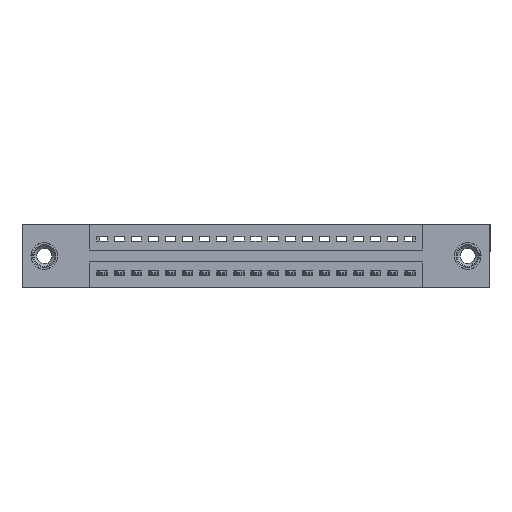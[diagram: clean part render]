
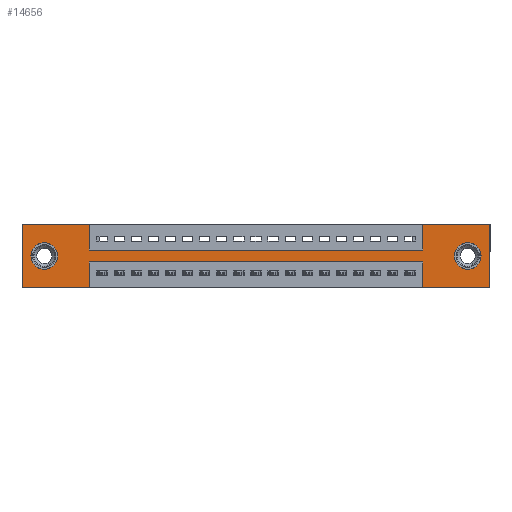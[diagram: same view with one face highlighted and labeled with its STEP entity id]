
A CAD part, front view. The second image highlights one B-rep face of the part: STEP entity #14656.
In plain terms, the highlighted planar face has unit normal (0, -1, 0).
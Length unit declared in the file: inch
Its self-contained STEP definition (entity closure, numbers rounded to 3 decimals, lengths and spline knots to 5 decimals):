
#80 = CARTESIAN_POINT ( 'NONE',  ( 0., 0., 0. ) ) ;
#273 = EDGE_CURVE ( 'NONE', #2156, #12889, #7085, .T. ) ;
#484 = ORIENTED_EDGE ( 'NONE', *, *, #7590, .F. ) ;
#587 = VECTOR ( 'NONE', #12232, 39.37008 ) ;
#705 = AXIS2_PLACEMENT_3D ( 'NONE', #14344, #5183, #9753 ) ;
#764 = CARTESIAN_POINT ( 'NONE',  ( 0.13, 0., -0.107 ) ) ;
#942 = VECTOR ( 'NONE', #14525, 39.37008 ) ;
#1250 = VECTOR ( 'NONE', #10655, 39.37008 ) ;
#1384 = CARTESIAN_POINT ( 'NONE',  ( 0.13, 0., -0.185 ) ) ;
#1507 = DIRECTION ( 'NONE',  ( 0., 1., 0. ) ) ;
#1546 = CARTESIAN_POINT ( 'NONE',  ( 0., 0., 0. ) ) ;
#1568 = ORIENTED_EDGE ( 'NONE', *, *, #5606, .F. ) ;
#1575 = ORIENTED_EDGE ( 'NONE', *, *, #3872, .F. ) ;
#1756 = ORIENTED_EDGE ( 'NONE', *, *, #2235, .T. ) ;
#1924 = CARTESIAN_POINT ( 'NONE',  ( 0.3925, 0., 0. ) ) ;
#1944 = VERTEX_POINT ( 'NONE', #3191 ) ;
#1962 = ORIENTED_EDGE ( 'NONE', *, *, #273, .F. ) ;
#2027 = LINE ( 'NONE', #11037, #2690 ) ;
#2156 = VERTEX_POINT ( 'NONE', #8819 ) ;
#2235 = EDGE_CURVE ( 'NONE', #10011, #6532, #18447, .T. ) ;
#2266 = FACE_BOUND ( 'NONE', #15954, .T. ) ;
#2497 = EDGE_LOOP ( 'NONE', ( #3591, #1756 ) ) ;
#2690 = VECTOR ( 'NONE', #15752, 39.37008 ) ;
#2843 = CARTESIAN_POINT ( 'NONE',  ( 0.13, 0., -0.263 ) ) ;
#3062 = DIRECTION ( 'NONE',  ( 0., 0., -1. ) ) ;
#3191 = CARTESIAN_POINT ( 'NONE',  ( 2.3425, 0., -0.37 ) ) ;
#3228 = LINE ( 'NONE', #9522, #13664 ) ;
#3409 = CARTESIAN_POINT ( 'NONE',  ( 0., 0., 0. ) ) ;
#3501 = CARTESIAN_POINT ( 'NONE',  ( 0.3925, 0., -0.22 ) ) ;
#3530 = DIRECTION ( 'NONE',  ( 0., 0., -1. ) ) ;
#3554 = CARTESIAN_POINT ( 'NONE',  ( 2.3425, 0., -0.22 ) ) ;
#3591 = ORIENTED_EDGE ( 'NONE', *, *, #18107, .T. ) ;
#3616 = ORIENTED_EDGE ( 'NONE', *, *, #11056, .F. ) ;
#3793 = AXIS2_PLACEMENT_3D ( 'NONE', #13927, #7788, #18443 ) ;
#3868 = LINE ( 'NONE', #17785, #5732 ) ;
#3872 = EDGE_CURVE ( 'NONE', #16847, #8612, #2027, .T. ) ;
#4174 = EDGE_CURVE ( 'NONE', #12920, #9953, #19240, .T. ) ;
#4819 = DIRECTION ( 'NONE',  ( -1., 0., 0. ) ) ;
#5183 = DIRECTION ( 'NONE',  ( 0., 1., 0. ) ) ;
#5366 = CARTESIAN_POINT ( 'NONE',  ( 2.735, 0., 0. ) ) ;
#5381 = VERTEX_POINT ( 'NONE', #764 ) ;
#5606 = EDGE_CURVE ( 'NONE', #9953, #2156, #18766, .T. ) ;
#5732 = VECTOR ( 'NONE', #19276, 39.37008 ) ;
#5865 = VECTOR ( 'NONE', #8054, 39.37008 ) ;
#5976 = CIRCLE ( 'NONE', #3793, 0.078 ) ;
#5977 = VECTOR ( 'NONE', #3062, 39.37008 ) ;
#5986 = VERTEX_POINT ( 'NONE', #2843 ) ;
#6260 = VECTOR ( 'NONE', #3530, 39.37008 ) ;
#6328 = EDGE_CURVE ( 'NONE', #5986, #5381, #8030, .T. ) ;
#6339 = LINE ( 'NONE', #18823, #10898 ) ;
#6477 = VERTEX_POINT ( 'NONE', #8709 ) ;
#6479 = ORIENTED_EDGE ( 'NONE', *, *, #13541, .F. ) ;
#6532 = VERTEX_POINT ( 'NONE', #10853 ) ;
#6617 = AXIS2_PLACEMENT_3D ( 'NONE', #16833, #10727, #10925 ) ;
#6768 = CIRCLE ( 'NONE', #705, 0.078 ) ;
#6853 = CARTESIAN_POINT ( 'NONE',  ( 2.735, 0., -0.37 ) ) ;
#7085 = LINE ( 'NONE', #1546, #1250 ) ;
#7575 = CARTESIAN_POINT ( 'NONE',  ( 0.3925, 0., 0. ) ) ;
#7590 = EDGE_CURVE ( 'NONE', #12889, #12862, #9896, .T. ) ;
#7725 = DIRECTION ( 'NONE',  ( 0., 0., 1. ) ) ;
#7788 = DIRECTION ( 'NONE',  ( 0., 1., 0. ) ) ;
#7964 = EDGE_CURVE ( 'NONE', #5381, #5986, #6768, .T. ) ;
#8030 = CIRCLE ( 'NONE', #16218, 0.078 ) ;
#8054 = DIRECTION ( 'NONE',  ( 1., 0., 0. ) ) ;
#8193 = CARTESIAN_POINT ( 'NONE',  ( 2.735, 0., 0. ) ) ;
#8194 = ORIENTED_EDGE ( 'NONE', *, *, #16904, .F. ) ;
#8229 = CARTESIAN_POINT ( 'NONE',  ( 2.605, 0., -0.263 ) ) ;
#8612 = VERTEX_POINT ( 'NONE', #3501 ) ;
#8709 = CARTESIAN_POINT ( 'NONE',  ( 0., 0., -0.37 ) ) ;
#8819 = CARTESIAN_POINT ( 'NONE',  ( 2.3425, 0., 0. ) ) ;
#8865 = CARTESIAN_POINT ( 'NONE',  ( 2.3425, 0., 0. ) ) ;
#9311 = ORIENTED_EDGE ( 'NONE', *, *, #7964, .T. ) ;
#9505 = PLANE ( 'NONE',  #10484 ) ;
#9522 = CARTESIAN_POINT ( 'NONE',  ( 0., 0., -0.37 ) ) ;
#9753 = DIRECTION ( 'NONE',  ( 0., 0., 1. ) ) ;
#9896 = LINE ( 'NONE', #8193, #942 ) ;
#9931 = DIRECTION ( 'NONE',  ( -1., 0., 0. ) ) ;
#9953 = VERTEX_POINT ( 'NONE', #18920 ) ;
#10011 = VERTEX_POINT ( 'NONE', #8229 ) ;
#10484 = AXIS2_PLACEMENT_3D ( 'NONE', #11036, #17357, #12561 ) ;
#10655 = DIRECTION ( 'NONE',  ( 1., 0., 0. ) ) ;
#10727 = DIRECTION ( 'NONE',  ( 0., 1., 0. ) ) ;
#10734 = CARTESIAN_POINT ( 'NONE',  ( 0.3925, 0., -0.15 ) ) ;
#10853 = CARTESIAN_POINT ( 'NONE',  ( 2.605, 0., -0.107 ) ) ;
#10856 = EDGE_CURVE ( 'NONE', #18356, #6477, #6339, .T. ) ;
#10898 = VECTOR ( 'NONE', #9931, 39.37008 ) ;
#10925 = DIRECTION ( 'NONE',  ( 0., 0., -1. ) ) ;
#11036 = CARTESIAN_POINT ( 'NONE',  ( 0., 0., -0.37 ) ) ;
#11037 = CARTESIAN_POINT ( 'NONE',  ( 0.3925, 0., -0.22 ) ) ;
#11056 = EDGE_CURVE ( 'NONE', #16878, #18790, #15141, .T. ) ;
#11195 = CARTESIAN_POINT ( 'NONE',  ( 0.3925, 0., -0.37 ) ) ;
#11761 = ORIENTED_EDGE ( 'NONE', *, *, #6328, .T. ) ;
#11988 = DIRECTION ( 'NONE',  ( 0., 0., 1. ) ) ;
#12232 = DIRECTION ( 'NONE',  ( 1., 0., 0. ) ) ;
#12561 = DIRECTION ( 'NONE',  ( 0., 0., -1. ) ) ;
#12862 = VERTEX_POINT ( 'NONE', #6853 ) ;
#12889 = VERTEX_POINT ( 'NONE', #5366 ) ;
#12920 = VERTEX_POINT ( 'NONE', #16102 ) ;
#13541 = EDGE_CURVE ( 'NONE', #18790, #12920, #17892, .T. ) ;
#13664 = VECTOR ( 'NONE', #4819, 39.37008 ) ;
#13927 = CARTESIAN_POINT ( 'NONE',  ( 2.605, 0., -0.185 ) ) ;
#14001 = EDGE_CURVE ( 'NONE', #1944, #16847, #3868, .T. ) ;
#14149 = LINE ( 'NONE', #11195, #6260 ) ;
#14344 = CARTESIAN_POINT ( 'NONE',  ( 0.13, 0., -0.185 ) ) ;
#14525 = DIRECTION ( 'NONE',  ( 0., 0., -1. ) ) ;
#14564 = ORIENTED_EDGE ( 'NONE', *, *, #18740, .F. ) ;
#14656 = ADVANCED_FACE ( 'NONE', ( #14782, #2266, #17874 ), #9505, .T. ) ;
#14782 = FACE_BOUND ( 'NONE', #2497, .T. ) ;
#14803 = DIRECTION ( 'NONE',  ( 0., 0., 1. ) ) ;
#15141 = LINE ( 'NONE', #16013, #5865 ) ;
#15752 = DIRECTION ( 'NONE',  ( -1., 0., 0. ) ) ;
#15954 = EDGE_LOOP ( 'NONE', ( #9311, #11761 ) ) ;
#16013 = CARTESIAN_POINT ( 'NONE',  ( 0., 0., 0. ) ) ;
#16096 = EDGE_LOOP ( 'NONE', ( #16782, #1575, #17666, #8194, #484, #1962, #1568, #18524, #6479, #3616, #14564, #17208 ) ) ;
#16102 = CARTESIAN_POINT ( 'NONE',  ( 0.3925, 0., -0.15 ) ) ;
#16218 = AXIS2_PLACEMENT_3D ( 'NONE', #1384, #1507, #11988 ) ;
#16646 = LINE ( 'NONE', #3409, #19002 ) ;
#16743 = EDGE_CURVE ( 'NONE', #8612, #18356, #14149, .T. ) ;
#16782 = ORIENTED_EDGE ( 'NONE', *, *, #16743, .F. ) ;
#16833 = CARTESIAN_POINT ( 'NONE',  ( 2.605, 0., -0.185 ) ) ;
#16847 = VERTEX_POINT ( 'NONE', #3554 ) ;
#16878 = VERTEX_POINT ( 'NONE', #80 ) ;
#16904 = EDGE_CURVE ( 'NONE', #12862, #1944, #3228, .T. ) ;
#17208 = ORIENTED_EDGE ( 'NONE', *, *, #10856, .F. ) ;
#17357 = DIRECTION ( 'NONE',  ( 0., -1., 0. ) ) ;
#17666 = ORIENTED_EDGE ( 'NONE', *, *, #14001, .F. ) ;
#17785 = CARTESIAN_POINT ( 'NONE',  ( 2.3425, 0., -0.37 ) ) ;
#17874 = FACE_OUTER_BOUND ( 'NONE', #16096, .T. ) ;
#17892 = LINE ( 'NONE', #7575, #5977 ) ;
#18107 = EDGE_CURVE ( 'NONE', #6532, #10011, #5976, .T. ) ;
#18356 = VERTEX_POINT ( 'NONE', #19372 ) ;
#18443 = DIRECTION ( 'NONE',  ( 0., 0., -1. ) ) ;
#18447 = CIRCLE ( 'NONE', #6617, 0.078 ) ;
#18524 = ORIENTED_EDGE ( 'NONE', *, *, #4174, .F. ) ;
#18740 = EDGE_CURVE ( 'NONE', #6477, #16878, #16646, .T. ) ;
#18766 = LINE ( 'NONE', #8865, #19443 ) ;
#18790 = VERTEX_POINT ( 'NONE', #1924 ) ;
#18823 = CARTESIAN_POINT ( 'NONE',  ( 0., 0., -0.37 ) ) ;
#18920 = CARTESIAN_POINT ( 'NONE',  ( 2.3425, 0., -0.15 ) ) ;
#19002 = VECTOR ( 'NONE', #7725, 39.37008 ) ;
#19240 = LINE ( 'NONE', #10734, #587 ) ;
#19276 = DIRECTION ( 'NONE',  ( 0., 0., 1. ) ) ;
#19372 = CARTESIAN_POINT ( 'NONE',  ( 0.3925, 0., -0.37 ) ) ;
#19443 = VECTOR ( 'NONE', #14803, 39.37008 ) ;
